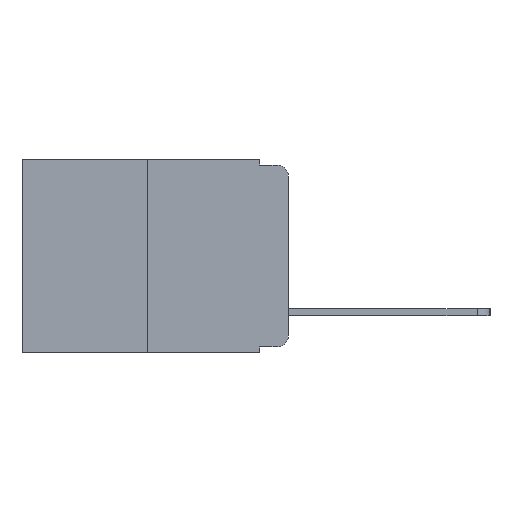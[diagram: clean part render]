
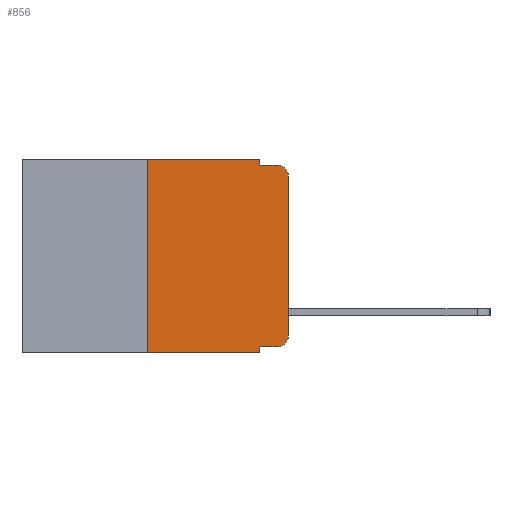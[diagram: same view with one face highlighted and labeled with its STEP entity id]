
A CAD part, left-side view. The second image highlights one B-rep face of the part: STEP entity #856.
In plain terms, the highlighted planar face has unit normal (-1, 0, 0).
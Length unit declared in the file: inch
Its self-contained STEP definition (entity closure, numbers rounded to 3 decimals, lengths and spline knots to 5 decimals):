
#5 = EDGE_CURVE ( 'NONE', #4696, #2340, #11205, .T. ) ;
#132 = CARTESIAN_POINT ( 'NONE',  ( 0., 0.051, -0.01 ) ) ;
#239 = LINE ( 'NONE', #4691, #6105 ) ;
#415 = DIRECTION ( 'NONE',  ( 0., 0., -1. ) ) ;
#421 = EDGE_CURVE ( 'NONE', #2678, #11553, #1637, .T. ) ;
#728 = AXIS2_PLACEMENT_3D ( 'NONE', #4395, #11117, #14208 ) ;
#856 = ADVANCED_FACE ( 'NONE', ( #8541 ), #12607, .F. ) ;
#1190 = EDGE_LOOP ( 'NONE', ( #4231, #1641, #5441, #7543, #9471, #9125, #8852, #5044, #10608, #12851 ) ) ;
#1637 = LINE ( 'NONE', #8575, #13514 ) ;
#1641 = ORIENTED_EDGE ( 'NONE', *, *, #6778, .T. ) ;
#1698 = AXIS2_PLACEMENT_3D ( 'NONE', #11596, #4759, #12741 ) ;
#1725 = CARTESIAN_POINT ( 'NONE',  ( 0., 0.051, -0.333 ) ) ;
#1769 = CARTESIAN_POINT ( 'NONE',  ( 0., 0.25, 0. ) ) ;
#1868 = VERTEX_POINT ( 'NONE', #14074 ) ;
#2018 = LINE ( 'NONE', #14298, #8216 ) ;
#2047 = DIRECTION ( 'NONE',  ( 0., -1., 0. ) ) ;
#2340 = VERTEX_POINT ( 'NONE', #3298 ) ;
#2671 = LINE ( 'NONE', #11264, #8480 ) ;
#2678 = VERTEX_POINT ( 'NONE', #14058 ) ;
#3083 = DIRECTION ( 'NONE',  ( 0., 0., -1. ) ) ;
#3099 = VERTEX_POINT ( 'NONE', #132 ) ;
#3298 = CARTESIAN_POINT ( 'NONE',  ( 0., 0.02, -0.333 ) ) ;
#4195 = VERTEX_POINT ( 'NONE', #10480 ) ;
#4231 = ORIENTED_EDGE ( 'NONE', *, *, #421, .T. ) ;
#4282 = AXIS2_PLACEMENT_3D ( 'NONE', #14211, #7419, #415 ) ;
#4323 = CARTESIAN_POINT ( 'NONE',  ( 0., 0.051, 0. ) ) ;
#4395 = CARTESIAN_POINT ( 'NONE',  ( 0., 0.473, 0. ) ) ;
#4612 = VERTEX_POINT ( 'NONE', #4323 ) ;
#4675 = VECTOR ( 'NONE', #11295, 39.37008 ) ;
#4691 = CARTESIAN_POINT ( 'NONE',  ( 0., 0.051, 0. ) ) ;
#4696 = VERTEX_POINT ( 'NONE', #7986 ) ;
#4759 = DIRECTION ( 'NONE',  ( -1., 0., 0. ) ) ;
#4959 = CARTESIAN_POINT ( 'NONE',  ( 0., 0.25, -0.343 ) ) ;
#5044 = ORIENTED_EDGE ( 'NONE', *, *, #7356, .F. ) ;
#5172 = VECTOR ( 'NONE', #3083, 39.37008 ) ;
#5441 = ORIENTED_EDGE ( 'NONE', *, *, #8975, .F. ) ;
#5570 = CIRCLE ( 'NONE', #1698, 0.02 ) ;
#5689 = DIRECTION ( 'NONE',  ( 0., -1., 0. ) ) ;
#6105 = VECTOR ( 'NONE', #9347, 39.37008 ) ;
#6593 = EDGE_CURVE ( 'NONE', #11184, #1868, #8117, .T. ) ;
#6727 = CARTESIAN_POINT ( 'NONE',  ( 0., 0.02, -0.01 ) ) ;
#6778 = EDGE_CURVE ( 'NONE', #11553, #14330, #5570, .T. ) ;
#6836 = CARTESIAN_POINT ( 'NONE',  ( 0., 0., -0.03 ) ) ;
#7356 = EDGE_CURVE ( 'NONE', #4696, #1868, #239, .T. ) ;
#7419 = DIRECTION ( 'NONE',  ( -1., 0., 0. ) ) ;
#7543 = ORIENTED_EDGE ( 'NONE', *, *, #7635, .F. ) ;
#7635 = EDGE_CURVE ( 'NONE', #4612, #3099, #12310, .T. ) ;
#7986 = CARTESIAN_POINT ( 'NONE',  ( 0., 0.051, -0.333 ) ) ;
#8117 = LINE ( 'NONE', #12390, #4675 ) ;
#8216 = VECTOR ( 'NONE', #13160, 39.37008 ) ;
#8217 = VECTOR ( 'NONE', #5689, 39.37008 ) ;
#8480 = VECTOR ( 'NONE', #2047, 39.37008 ) ;
#8541 = FACE_OUTER_BOUND ( 'NONE', #1190, .T. ) ;
#8575 = CARTESIAN_POINT ( 'NONE',  ( 0., 0., 0. ) ) ;
#8852 = ORIENTED_EDGE ( 'NONE', *, *, #6593, .T. ) ;
#8975 = EDGE_CURVE ( 'NONE', #3099, #14330, #2018, .T. ) ;
#9125 = ORIENTED_EDGE ( 'NONE', *, *, #13713, .F. ) ;
#9347 = DIRECTION ( 'NONE',  ( 0., 0., -1. ) ) ;
#9471 = ORIENTED_EDGE ( 'NONE', *, *, #13227, .F. ) ;
#10480 = CARTESIAN_POINT ( 'NONE',  ( 0., 0.25, 0. ) ) ;
#10608 = ORIENTED_EDGE ( 'NONE', *, *, #5, .T. ) ;
#11117 = DIRECTION ( 'NONE',  ( 1., 0., 0. ) ) ;
#11184 = VERTEX_POINT ( 'NONE', #4959 ) ;
#11205 = LINE ( 'NONE', #1725, #8217 ) ;
#11264 = CARTESIAN_POINT ( 'NONE',  ( 0., 0.473, 0. ) ) ;
#11295 = DIRECTION ( 'NONE',  ( 0., -1., 0. ) ) ;
#11553 = VERTEX_POINT ( 'NONE', #6836 ) ;
#11596 = CARTESIAN_POINT ( 'NONE',  ( 0., 0.02, -0.03 ) ) ;
#11640 = VECTOR ( 'NONE', #14387, 39.37008 ) ;
#11990 = LINE ( 'NONE', #1769, #11640 ) ;
#12310 = LINE ( 'NONE', #13377, #5172 ) ;
#12377 = CIRCLE ( 'NONE', #4282, 0.02 ) ;
#12390 = CARTESIAN_POINT ( 'NONE',  ( 0., 0.473, -0.343 ) ) ;
#12607 = PLANE ( 'NONE',  #728 ) ;
#12741 = DIRECTION ( 'NONE',  ( 0., 0., -1. ) ) ;
#12851 = ORIENTED_EDGE ( 'NONE', *, *, #12955, .T. ) ;
#12955 = EDGE_CURVE ( 'NONE', #2340, #2678, #12377, .T. ) ;
#13160 = DIRECTION ( 'NONE',  ( 0., -1., 0. ) ) ;
#13227 = EDGE_CURVE ( 'NONE', #4195, #4612, #2671, .T. ) ;
#13377 = CARTESIAN_POINT ( 'NONE',  ( 0., 0.051, 0. ) ) ;
#13514 = VECTOR ( 'NONE', #14414, 39.37008 ) ;
#13713 = EDGE_CURVE ( 'NONE', #11184, #4195, #11990, .T. ) ;
#14058 = CARTESIAN_POINT ( 'NONE',  ( 0., 0., -0.313 ) ) ;
#14074 = CARTESIAN_POINT ( 'NONE',  ( 0., 0.051, -0.343 ) ) ;
#14208 = DIRECTION ( 'NONE',  ( 0., 0., -1. ) ) ;
#14211 = CARTESIAN_POINT ( 'NONE',  ( 0., 0.02, -0.313 ) ) ;
#14298 = CARTESIAN_POINT ( 'NONE',  ( 0., 0.051, -0.01 ) ) ;
#14330 = VERTEX_POINT ( 'NONE', #6727 ) ;
#14387 = DIRECTION ( 'NONE',  ( 0., 0., 1. ) ) ;
#14414 = DIRECTION ( 'NONE',  ( 0., 0., 1. ) ) ;
